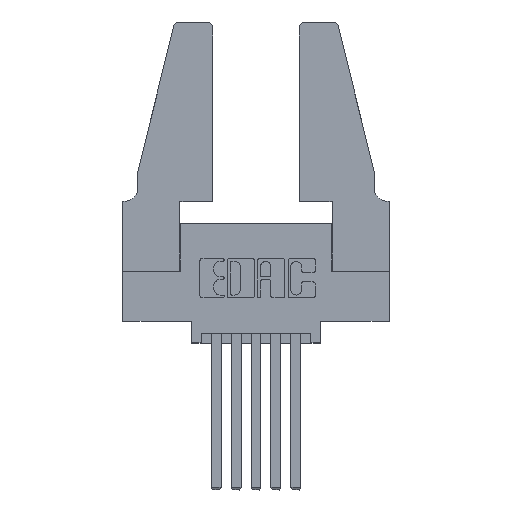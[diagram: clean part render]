
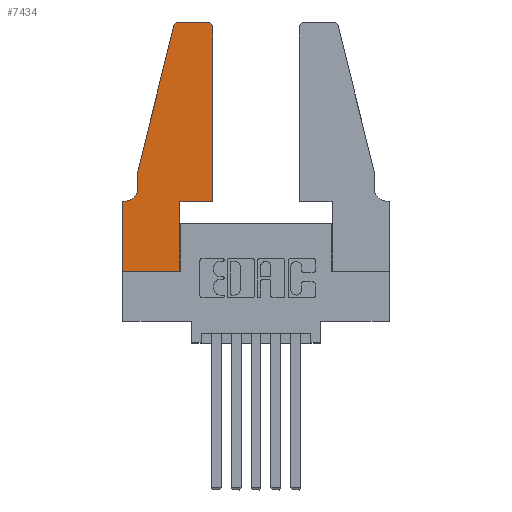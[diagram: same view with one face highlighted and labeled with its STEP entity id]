
A CAD part, top view. The second image highlights one B-rep face of the part: STEP entity #7434.
In plain terms, the highlighted planar face has unit normal (0, 0, 1).
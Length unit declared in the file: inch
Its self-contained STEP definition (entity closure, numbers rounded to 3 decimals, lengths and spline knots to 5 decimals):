
#82 = VERTEX_POINT ( 'NONE', #494 ) ;
#109 = ORIENTED_EDGE ( 'NONE', *, *, #3723, .T. ) ;
#156 = ORIENTED_EDGE ( 'NONE', *, *, #10381, .T. ) ;
#259 = VECTOR ( 'NONE', #1526, 39.37008 ) ;
#287 = LINE ( 'NONE', #10234, #600 ) ;
#328 = DIRECTION ( 'NONE',  ( -1., 0., 0. ) ) ;
#392 = VECTOR ( 'NONE', #8401, 39.37008 ) ;
#419 = ORIENTED_EDGE ( 'NONE', *, *, #5883, .T. ) ;
#491 = DIRECTION ( 'NONE',  ( 0., 0., 1. ) ) ;
#494 = CARTESIAN_POINT ( 'NONE',  ( 0.25487, 1.22718, 0.37 ) ) ;
#586 = CARTESIAN_POINT ( 'NONE',  ( 0.0755, 0.5, 0.37 ) ) ;
#600 = VECTOR ( 'NONE', #6151, 39.37008 ) ;
#697 = CARTESIAN_POINT ( 'NONE',  ( 0.4505, 0.35, 0.37 ) ) ;
#1126 = ORIENTED_EDGE ( 'NONE', *, *, #10465, .T. ) ;
#1333 = VERTEX_POINT ( 'NONE', #4477 ) ;
#1479 = AXIS2_PLACEMENT_3D ( 'NONE', #1568, #7521, #2493 ) ;
#1526 = DIRECTION ( 'NONE',  ( -0.239, -0.971, 0. ) ) ;
#1568 = CARTESIAN_POINT ( 'NONE',  ( 0.284, 1.22, 0.37 ) ) ;
#1623 = VERTEX_POINT ( 'NONE', #10788 ) ;
#1761 = CARTESIAN_POINT ( 'NONE',  ( 0.0755, 0.42, 0.37 ) ) ;
#1787 = LINE ( 'NONE', #10502, #3847 ) ;
#1956 = DIRECTION ( 'NONE',  ( 0., -1., 0. ) ) ;
#2028 = ORIENTED_EDGE ( 'NONE', *, *, #9740, .T. ) ;
#2050 = ORIENTED_EDGE ( 'NONE', *, *, #2438, .T. ) ;
#2285 = DIRECTION ( 'NONE',  ( -1., 0., 0. ) ) ;
#2286 = ORIENTED_EDGE ( 'NONE', *, *, #6880, .T. ) ;
#2438 = EDGE_CURVE ( 'NONE', #9204, #1623, #9755, .T. ) ;
#2493 = DIRECTION ( 'NONE',  ( 1., 0., 0. ) ) ;
#2555 = VECTOR ( 'NONE', #6984, 39.37008 ) ;
#2837 = AXIS2_PLACEMENT_3D ( 'NONE', #5722, #491, #6568 ) ;
#3156 = CIRCLE ( 'NONE', #8498, 0.07 ) ;
#3241 = VERTEX_POINT ( 'NONE', #4149 ) ;
#3516 = CARTESIAN_POINT ( 'NONE',  ( 0., 0., 0.37 ) ) ;
#3553 = LINE ( 'NONE', #4020, #9864 ) ;
#3723 = EDGE_CURVE ( 'NONE', #10428, #1333, #11005, .T. ) ;
#3781 = VERTEX_POINT ( 'NONE', #10119 ) ;
#3847 = VECTOR ( 'NONE', #328, 39.37008 ) ;
#3883 = CARTESIAN_POINT ( 'NONE',  ( 0.0055, 0.42, 0.37 ) ) ;
#4020 = CARTESIAN_POINT ( 'NONE',  ( 0.2605, 1.25, 0.37 ) ) ;
#4149 = CARTESIAN_POINT ( 'NONE',  ( 0.284, 1.25, 0.37 ) ) ;
#4381 = VERTEX_POINT ( 'NONE', #7548 ) ;
#4398 = EDGE_CURVE ( 'NONE', #1333, #10861, #7054, .T. ) ;
#4470 = CARTESIAN_POINT ( 'NONE',  ( 0.0755, 0.5, 0.37 ) ) ;
#4477 = CARTESIAN_POINT ( 'NONE',  ( 0.2865, 0.35, 0.37 ) ) ;
#4523 = ORIENTED_EDGE ( 'NONE', *, *, #9559, .T. ) ;
#4733 = DIRECTION ( 'NONE',  ( -1., 0., 0. ) ) ;
#4881 = VERTEX_POINT ( 'NONE', #8120 ) ;
#4897 = ORIENTED_EDGE ( 'NONE', *, *, #9048, .T. ) ;
#5360 = ORIENTED_EDGE ( 'NONE', *, *, #8499, .T. ) ;
#5502 = CARTESIAN_POINT ( 'NONE',  ( 0.4505, 0.35, 0.37 ) ) ;
#5722 = CARTESIAN_POINT ( 'NONE',  ( 0., 0.35, 0.37 ) ) ;
#5773 = CARTESIAN_POINT ( 'NONE',  ( 0.2865, 0., 0.37 ) ) ;
#5798 = LINE ( 'NONE', #6344, #9641 ) ;
#5831 = VERTEX_POINT ( 'NONE', #1761 ) ;
#5834 = AXIS2_PLACEMENT_3D ( 'NONE', #6386, #6734, #10407 ) ;
#5883 = EDGE_CURVE ( 'NONE', #3781, #5831, #9205, .T. ) ;
#6151 = DIRECTION ( 'NONE',  ( 0., 1., 0. ) ) ;
#6213 = CIRCLE ( 'NONE', #1479, 0.03 ) ;
#6316 = VECTOR ( 'NONE', #1956, 39.37008 ) ;
#6344 = CARTESIAN_POINT ( 'NONE',  ( 0., 0., 0.37 ) ) ;
#6349 = ORIENTED_EDGE ( 'NONE', *, *, #8968, .T. ) ;
#6386 = CARTESIAN_POINT ( 'NONE',  ( 0.4205, 1.22, 0.37 ) ) ;
#6568 = DIRECTION ( 'NONE',  ( 1., 0., 0. ) ) ;
#6734 = DIRECTION ( 'NONE',  ( 0., 0., 1. ) ) ;
#6880 = EDGE_CURVE ( 'NONE', #3241, #82, #6213, .T. ) ;
#6951 = LINE ( 'NONE', #586, #259 ) ;
#6984 = DIRECTION ( 'NONE',  ( 0., -1., 0. ) ) ;
#7054 = LINE ( 'NONE', #697, #392 ) ;
#7406 = CARTESIAN_POINT ( 'NONE',  ( 0.4505, 1.22, 0.37 ) ) ;
#7434 = ADVANCED_FACE ( 'NONE', ( #9300 ), #9772, .T. ) ;
#7521 = DIRECTION ( 'NONE',  ( 0., 0., 1. ) ) ;
#7548 = CARTESIAN_POINT ( 'NONE',  ( 0.0055, 0.35, 0.37 ) ) ;
#8120 = CARTESIAN_POINT ( 'NONE',  ( 0., 0.35, 0.37 ) ) ;
#8284 = EDGE_LOOP ( 'NONE', ( #156, #2286, #1126, #419, #2028, #5360, #6349, #4897, #109, #10589, #4523, #2050 ) ) ;
#8401 = DIRECTION ( 'NONE',  ( 1., 0., 0. ) ) ;
#8498 = AXIS2_PLACEMENT_3D ( 'NONE', #3883, #9653, #4733 ) ;
#8499 = EDGE_CURVE ( 'NONE', #4381, #4881, #1787, .T. ) ;
#8511 = LINE ( 'NONE', #10280, #6316 ) ;
#8852 = VECTOR ( 'NONE', #10276, 39.37008 ) ;
#8968 = EDGE_CURVE ( 'NONE', #4881, #10071, #8511, .T. ) ;
#9048 = EDGE_CURVE ( 'NONE', #10071, #10428, #5798, .T. ) ;
#9204 = VERTEX_POINT ( 'NONE', #7406 ) ;
#9205 = LINE ( 'NONE', #4470, #2555 ) ;
#9300 = FACE_OUTER_BOUND ( 'NONE', #8284, .T. ) ;
#9559 = EDGE_CURVE ( 'NONE', #10861, #9204, #287, .T. ) ;
#9601 = DIRECTION ( 'NONE',  ( 1., 0., 0. ) ) ;
#9641 = VECTOR ( 'NONE', #9601, 39.37008 ) ;
#9653 = DIRECTION ( 'NONE',  ( 0., 0., -1. ) ) ;
#9740 = EDGE_CURVE ( 'NONE', #5831, #4381, #3156, .T. ) ;
#9755 = CIRCLE ( 'NONE', #5834, 0.03 ) ;
#9772 = PLANE ( 'NONE',  #2837 ) ;
#9864 = VECTOR ( 'NONE', #2285, 39.37008 ) ;
#10071 = VERTEX_POINT ( 'NONE', #3516 ) ;
#10119 = CARTESIAN_POINT ( 'NONE',  ( 0.0755, 0.5, 0.37 ) ) ;
#10194 = CARTESIAN_POINT ( 'NONE',  ( 0.2865, 0.35, 0.37 ) ) ;
#10234 = CARTESIAN_POINT ( 'NONE',  ( 0.4505, 0.35, 0.37 ) ) ;
#10276 = DIRECTION ( 'NONE',  ( 0., 1., 0. ) ) ;
#10280 = CARTESIAN_POINT ( 'NONE',  ( 0., 0., 0.37 ) ) ;
#10381 = EDGE_CURVE ( 'NONE', #1623, #3241, #3553, .T. ) ;
#10407 = DIRECTION ( 'NONE',  ( 1., 0., 0. ) ) ;
#10428 = VERTEX_POINT ( 'NONE', #5773 ) ;
#10465 = EDGE_CURVE ( 'NONE', #82, #3781, #6951, .T. ) ;
#10502 = CARTESIAN_POINT ( 'NONE',  ( 0.0755, 0.35, 0.37 ) ) ;
#10589 = ORIENTED_EDGE ( 'NONE', *, *, #4398, .T. ) ;
#10788 = CARTESIAN_POINT ( 'NONE',  ( 0.4205, 1.25, 0.37 ) ) ;
#10861 = VERTEX_POINT ( 'NONE', #5502 ) ;
#11005 = LINE ( 'NONE', #10194, #8852 ) ;
